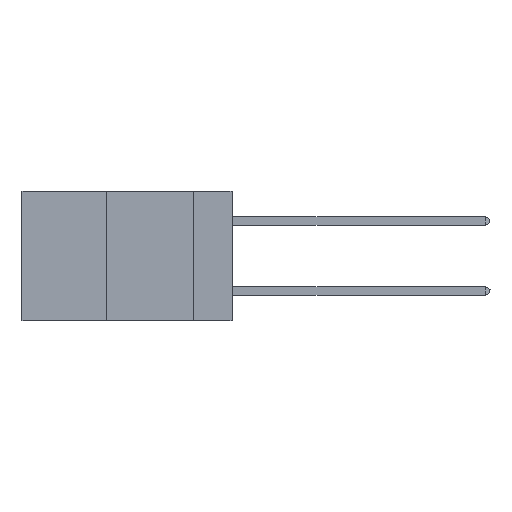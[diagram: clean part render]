
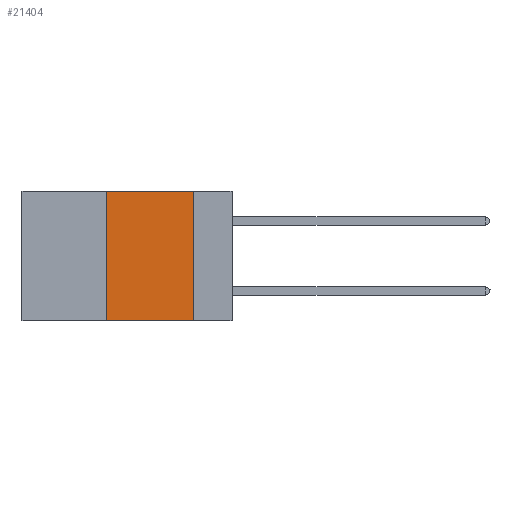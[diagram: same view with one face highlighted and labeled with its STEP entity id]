
A CAD part, left-side view. The second image highlights one B-rep face of the part: STEP entity #21404.
In plain terms, the highlighted planar face has unit normal (-1, 0, 0).
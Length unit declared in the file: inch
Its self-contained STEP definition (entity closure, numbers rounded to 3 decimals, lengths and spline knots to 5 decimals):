
#40 = EDGE_LOOP ( 'NONE', ( #20304, #2553, #7452, #13133 ) ) ;
#398 = CARTESIAN_POINT ( 'NONE',  ( 0., 0.11, 0. ) ) ;
#1151 = CARTESIAN_POINT ( 'NONE',  ( 0., 0.36, 0. ) ) ;
#1956 = PLANE ( 'NONE',  #14272 ) ;
#2212 = VERTEX_POINT ( 'NONE', #18987 ) ;
#2553 = ORIENTED_EDGE ( 'NONE', *, *, #24624, .F. ) ;
#4682 = DIRECTION ( 'NONE',  ( 0., 0., -1. ) ) ;
#5842 = EDGE_CURVE ( 'NONE', #2212, #17302, #19954, .T. ) ;
#6043 = VECTOR ( 'NONE', #15156, 39.37008 ) ;
#7452 = ORIENTED_EDGE ( 'NONE', *, *, #22759, .F. ) ;
#7627 = DIRECTION ( 'NONE',  ( 0., 0., -1. ) ) ;
#7849 = DIRECTION ( 'NONE',  ( 0., -1., 0. ) ) ;
#9500 = CARTESIAN_POINT ( 'NONE',  ( 0., 0.36, 0. ) ) ;
#9805 = VECTOR ( 'NONE', #17133, 39.37008 ) ;
#10479 = VERTEX_POINT ( 'NONE', #1151 ) ;
#11172 = LINE ( 'NONE', #9500, #6043 ) ;
#13133 = ORIENTED_EDGE ( 'NONE', *, *, #5842, .T. ) ;
#13292 = CARTESIAN_POINT ( 'NONE',  ( 0., 0.11, -0.37 ) ) ;
#13617 = CARTESIAN_POINT ( 'NONE',  ( 0., 0.6, 0. ) ) ;
#13726 = VECTOR ( 'NONE', #7849, 39.37008 ) ;
#14163 = CARTESIAN_POINT ( 'NONE',  ( 0., 0.11, 0. ) ) ;
#14272 = AXIS2_PLACEMENT_3D ( 'NONE', #15118, #15201, #7627 ) ;
#14301 = EDGE_CURVE ( 'NONE', #19756, #17302, #16917, .T. ) ;
#15118 = CARTESIAN_POINT ( 'NONE',  ( 0., 0.6, 0. ) ) ;
#15156 = DIRECTION ( 'NONE',  ( 0., 0., 1. ) ) ;
#15201 = DIRECTION ( 'NONE',  ( 1., 0., 0. ) ) ;
#16917 = LINE ( 'NONE', #14163, #21965 ) ;
#17133 = DIRECTION ( 'NONE',  ( 0., -1., 0. ) ) ;
#17302 = VERTEX_POINT ( 'NONE', #13292 ) ;
#18402 = CARTESIAN_POINT ( 'NONE',  ( 0., 0.6, -0.37 ) ) ;
#18987 = CARTESIAN_POINT ( 'NONE',  ( 0., 0.36, -0.37 ) ) ;
#18996 = FACE_OUTER_BOUND ( 'NONE', #40, .T. ) ;
#19756 = VERTEX_POINT ( 'NONE', #398 ) ;
#19954 = LINE ( 'NONE', #18402, #9805 ) ;
#20304 = ORIENTED_EDGE ( 'NONE', *, *, #14301, .F. ) ;
#20916 = LINE ( 'NONE', #13617, #13726 ) ;
#21404 = ADVANCED_FACE ( 'NONE', ( #18996 ), #1956, .F. ) ;
#21965 = VECTOR ( 'NONE', #4682, 39.37008 ) ;
#22759 = EDGE_CURVE ( 'NONE', #2212, #10479, #11172, .T. ) ;
#24624 = EDGE_CURVE ( 'NONE', #10479, #19756, #20916, .T. ) ;
